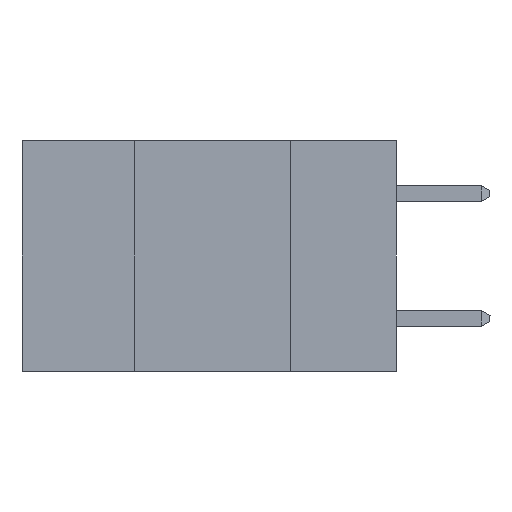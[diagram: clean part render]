
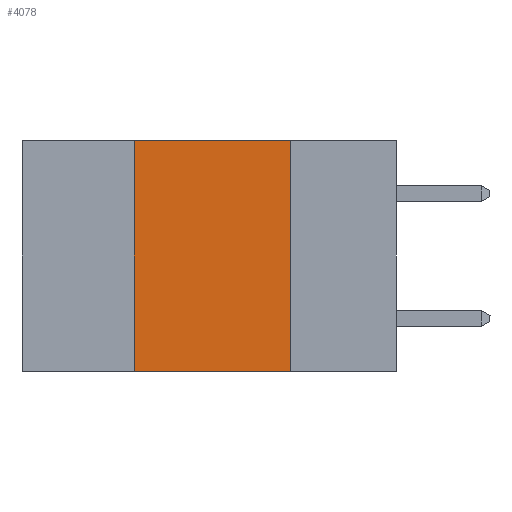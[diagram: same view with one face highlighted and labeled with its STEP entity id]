
A CAD part, left-side view. The second image highlights one B-rep face of the part: STEP entity #4078.
In plain terms, the highlighted planar face has unit normal (-1, 0, 0).
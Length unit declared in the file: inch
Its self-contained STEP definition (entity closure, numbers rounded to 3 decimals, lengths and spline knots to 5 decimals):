
#56 = EDGE_CURVE ( 'NONE', #12290, #7863, #4353, .T. ) ;
#373 = CARTESIAN_POINT ( 'NONE',  ( 0., 0.6, -0.37 ) ) ;
#441 = DIRECTION ( 'NONE',  ( 0., -1., 0. ) ) ;
#1015 = VERTEX_POINT ( 'NONE', #3151 ) ;
#1423 = VECTOR ( 'NONE', #7970, 39.37008 ) ;
#1460 = VECTOR ( 'NONE', #10929, 39.37008 ) ;
#2122 = LINE ( 'NONE', #7198, #4773 ) ;
#2432 = CARTESIAN_POINT ( 'NONE',  ( 0., 0.42, -0.37 ) ) ;
#3151 = CARTESIAN_POINT ( 'NONE',  ( 0., 0.42, 0. ) ) ;
#4078 = ADVANCED_FACE ( 'NONE', ( #8682 ), #8011, .F. ) ;
#4239 = VECTOR ( 'NONE', #441, 39.37008 ) ;
#4353 = LINE ( 'NONE', #4826, #1423 ) ;
#4615 = CARTESIAN_POINT ( 'NONE',  ( 0., 0.17, -0.37 ) ) ;
#4773 = VECTOR ( 'NONE', #6970, 39.37008 ) ;
#4826 = CARTESIAN_POINT ( 'NONE',  ( 0., 0.17, -0.37 ) ) ;
#5902 = EDGE_LOOP ( 'NONE', ( #8069, #8485, #8536, #8592 ) ) ;
#6970 = DIRECTION ( 'NONE',  ( 0., 0., 1. ) ) ;
#7198 = CARTESIAN_POINT ( 'NONE',  ( 0., 0.42, -0.37 ) ) ;
#7442 = DIRECTION ( 'NONE',  ( 0., 0., -1. ) ) ;
#7539 = DIRECTION ( 'NONE',  ( 1., 0., 0. ) ) ;
#7746 = CARTESIAN_POINT ( 'NONE',  ( 0., 0.6, 0. ) ) ;
#7863 = VERTEX_POINT ( 'NONE', #4615 ) ;
#7970 = DIRECTION ( 'NONE',  ( 0., 0., -1. ) ) ;
#8011 = PLANE ( 'NONE',  #10642 ) ;
#8069 = ORIENTED_EDGE ( 'NONE', *, *, #56, .F. ) ;
#8485 = ORIENTED_EDGE ( 'NONE', *, *, #12534, .F. ) ;
#8536 = ORIENTED_EDGE ( 'NONE', *, *, #11207, .F. ) ;
#8592 = ORIENTED_EDGE ( 'NONE', *, *, #10508, .T. ) ;
#8682 = FACE_OUTER_BOUND ( 'NONE', #5902, .T. ) ;
#10508 = EDGE_CURVE ( 'NONE', #12033, #7863, #10667, .T. ) ;
#10642 = AXIS2_PLACEMENT_3D ( 'NONE', #7746, #7539, #7442 ) ;
#10667 = LINE ( 'NONE', #373, #4239 ) ;
#10879 = CARTESIAN_POINT ( 'NONE',  ( 0., 0.6, 0. ) ) ;
#10929 = DIRECTION ( 'NONE',  ( 0., -1., 0. ) ) ;
#11207 = EDGE_CURVE ( 'NONE', #12033, #1015, #2122, .T. ) ;
#12033 = VERTEX_POINT ( 'NONE', #2432 ) ;
#12203 = LINE ( 'NONE', #10879, #1460 ) ;
#12290 = VERTEX_POINT ( 'NONE', #13129 ) ;
#12534 = EDGE_CURVE ( 'NONE', #1015, #12290, #12203, .T. ) ;
#13129 = CARTESIAN_POINT ( 'NONE',  ( 0., 0.17, 0. ) ) ;
